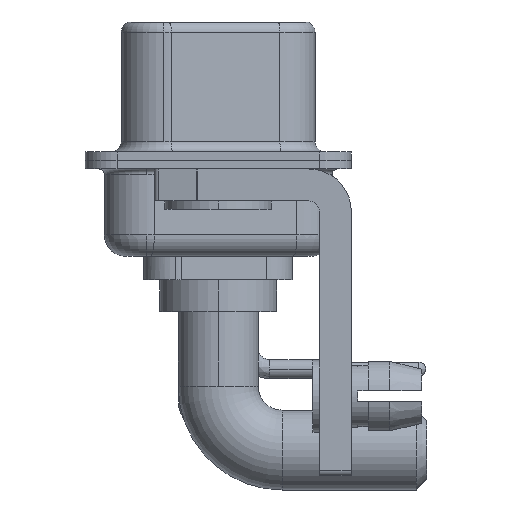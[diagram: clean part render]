
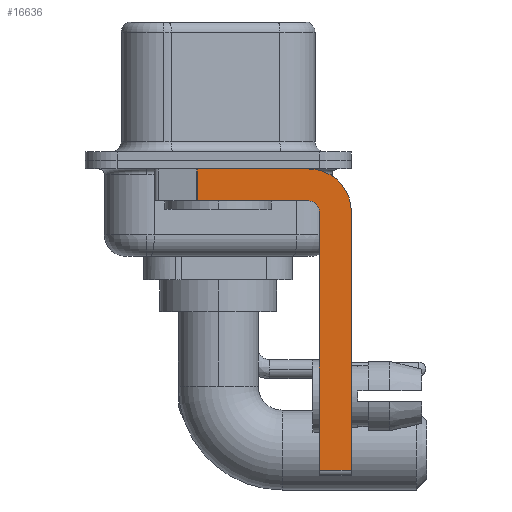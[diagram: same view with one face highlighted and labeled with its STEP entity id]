
A CAD part, left-side view. The second image highlights one B-rep face of the part: STEP entity #16636.
In plain terms, the highlighted planar face has unit normal (-1, 0, 0).
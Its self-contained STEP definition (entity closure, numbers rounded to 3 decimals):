
#253 = VECTOR ( 'NONE', #7380, 1000. ) ;
#586 = CARTESIAN_POINT ( 'NONE',  ( -2.9, -4.25, -1.9 ) ) ;
#667 = VECTOR ( 'NONE', #15237, 1000. ) ;
#1431 = CARTESIAN_POINT ( 'NONE',  ( -2.9, -4.75, -2.4 ) ) ;
#2130 = DIRECTION ( 'NONE',  ( 0., 0., -1. ) ) ;
#2554 = DIRECTION ( 'NONE',  ( 0., 0., 1. ) ) ;
#2866 = CARTESIAN_POINT ( 'NONE',  ( -2.9, 0.978, -1.9 ) ) ;
#2992 = CARTESIAN_POINT ( 'NONE',  ( -2.9, -4.25, -2.4 ) ) ;
#3238 = DIRECTION ( 'NONE',  ( 0., 0., -1. ) ) ;
#3446 = LINE ( 'NONE', #18892, #667 ) ;
#3705 = VECTOR ( 'NONE', #22889, 1000. ) ;
#5102 = VECTOR ( 'NONE', #16185, 1000. ) ;
#5731 = VERTEX_POINT ( 'NONE', #22492 ) ;
#5756 = VERTEX_POINT ( 'NONE', #24498 ) ;
#6227 = ORIENTED_EDGE ( 'NONE', *, *, #8527, .F. ) ;
#6578 = ORIENTED_EDGE ( 'NONE', *, *, #6787, .F. ) ;
#6787 = EDGE_CURVE ( 'NONE', #19102, #7643, #24356, .T. ) ;
#6796 = CARTESIAN_POINT ( 'NONE',  ( -2.9, -4.25, -0.4 ) ) ;
#6872 = DIRECTION ( 'NONE',  ( 1., 0., 0. ) ) ;
#7125 = CIRCLE ( 'NONE', #12734, 2. ) ;
#7166 = CARTESIAN_POINT ( 'NONE',  ( -2.9, -4.75, -14.55 ) ) ;
#7380 = DIRECTION ( 'NONE',  ( 0., 1., 0. ) ) ;
#7643 = VERTEX_POINT ( 'NONE', #24664 ) ;
#8155 = CARTESIAN_POINT ( 'NONE',  ( -2.9, -4.25, -2.4 ) ) ;
#8494 = EDGE_CURVE ( 'NONE', #5731, #7643, #18432, .T. ) ;
#8527 = EDGE_CURVE ( 'NONE', #14508, #23129, #7125, .T. ) ;
#8958 = VERTEX_POINT ( 'NONE', #1431 ) ;
#9552 = LINE ( 'NONE', #11188, #3705 ) ;
#9777 = EDGE_CURVE ( 'NONE', #5731, #14508, #16313, .T. ) ;
#10339 = LINE ( 'NONE', #16367, #10502 ) ;
#10502 = VECTOR ( 'NONE', #2554, 1000. ) ;
#10535 = CARTESIAN_POINT ( 'NONE',  ( -2.9, -6.25, -2.4 ) ) ;
#11188 = CARTESIAN_POINT ( 'NONE',  ( -2.9, -4.25, -14.55 ) ) ;
#12651 = CARTESIAN_POINT ( 'NONE',  ( -2.9, 3., -0.4 ) ) ;
#12734 = AXIS2_PLACEMENT_3D ( 'NONE', #2992, #6872, #3238 ) ;
#13064 = DIRECTION ( 'NONE',  ( -1., 0., 0. ) ) ;
#13166 = VECTOR ( 'NONE', #16558, 1000. ) ;
#14423 = EDGE_LOOP ( 'NONE', ( #16353, #18443, #6578, #16336, #24574, #15746, #21091, #6227 ) ) ;
#14508 = VERTEX_POINT ( 'NONE', #6796 ) ;
#14820 = EDGE_CURVE ( 'NONE', #19154, #5756, #9552, .T. ) ;
#15237 = DIRECTION ( 'NONE',  ( 0., 0., -1. ) ) ;
#15746 = ORIENTED_EDGE ( 'NONE', *, *, #14820, .T. ) ;
#15810 = DIRECTION ( 'NONE',  ( 1., 0., 0. ) ) ;
#16055 = FACE_OUTER_BOUND ( 'NONE', #14423, .T. ) ;
#16185 = DIRECTION ( 'NONE',  ( 0., 0., -1. ) ) ;
#16313 = LINE ( 'NONE', #12651, #13166 ) ;
#16336 = ORIENTED_EDGE ( 'NONE', *, *, #21153, .F. ) ;
#16353 = ORIENTED_EDGE ( 'NONE', *, *, #9777, .F. ) ;
#16367 = CARTESIAN_POINT ( 'NONE',  ( -2.9, -4.75, -14.8 ) ) ;
#16558 = DIRECTION ( 'NONE',  ( 0., -1., 0. ) ) ;
#16636 = ADVANCED_FACE ( 'NONE', ( #16055 ), #17446, .F. ) ;
#17446 = PLANE ( 'NONE',  #19708 ) ;
#17695 = EDGE_CURVE ( 'NONE', #19154, #8958, #10339, .T. ) ;
#18432 = LINE ( 'NONE', #2866, #5102 ) ;
#18443 = ORIENTED_EDGE ( 'NONE', *, *, #8494, .T. ) ;
#18892 = CARTESIAN_POINT ( 'NONE',  ( -2.9, -6.25, -2.4 ) ) ;
#19102 = VERTEX_POINT ( 'NONE', #586 ) ;
#19154 = VERTEX_POINT ( 'NONE', #7166 ) ;
#19708 = AXIS2_PLACEMENT_3D ( 'NONE', #8155, #15810, #2130 ) ;
#20742 = DIRECTION ( 'NONE',  ( 0., 0., 1. ) ) ;
#21091 = ORIENTED_EDGE ( 'NONE', *, *, #24631, .F. ) ;
#21153 = EDGE_CURVE ( 'NONE', #8958, #19102, #23052, .T. ) ;
#22492 = CARTESIAN_POINT ( 'NONE',  ( -2.9, 0.978, -0.4 ) ) ;
#22889 = DIRECTION ( 'NONE',  ( 0., -1., 0. ) ) ;
#23052 = CIRCLE ( 'NONE', #24647, 0.5 ) ;
#23129 = VERTEX_POINT ( 'NONE', #10535 ) ;
#23231 = CARTESIAN_POINT ( 'NONE',  ( -2.9, -4.25, -2.4 ) ) ;
#24356 = LINE ( 'NONE', #24603, #253 ) ;
#24498 = CARTESIAN_POINT ( 'NONE',  ( -2.9, -6.25, -14.55 ) ) ;
#24574 = ORIENTED_EDGE ( 'NONE', *, *, #17695, .F. ) ;
#24603 = CARTESIAN_POINT ( 'NONE',  ( -2.9, -4.25, -1.9 ) ) ;
#24631 = EDGE_CURVE ( 'NONE', #23129, #5756, #3446, .T. ) ;
#24647 = AXIS2_PLACEMENT_3D ( 'NONE', #23231, #13064, #20742 ) ;
#24664 = CARTESIAN_POINT ( 'NONE',  ( -2.9, 0.978, -1.9 ) ) ;
